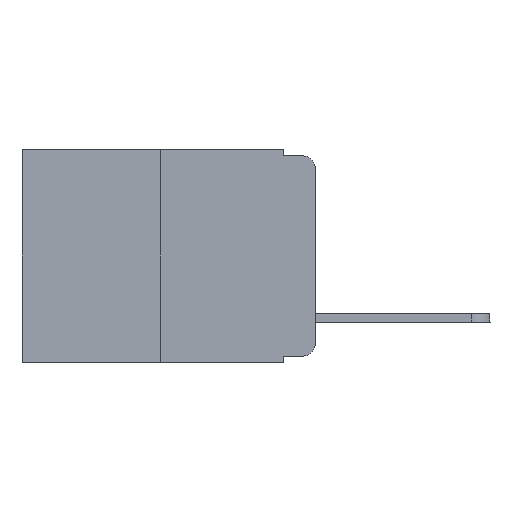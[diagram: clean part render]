
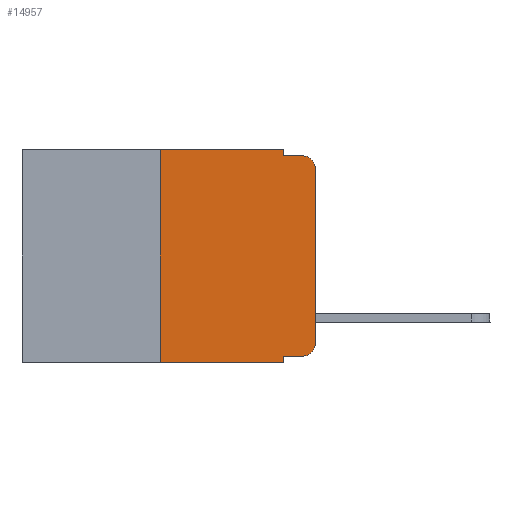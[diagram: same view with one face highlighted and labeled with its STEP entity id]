
A CAD part, left-side view. The second image highlights one B-rep face of the part: STEP entity #14957.
In plain terms, the highlighted planar face has unit normal (-1, 0, 0).
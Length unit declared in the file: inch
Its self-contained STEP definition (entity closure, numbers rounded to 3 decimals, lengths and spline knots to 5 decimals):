
#62 = DIRECTION ( 'NONE',  ( -1., 0., 0. ) ) ;
#193 = VECTOR ( 'NONE', #1713, 39.37008 ) ;
#206 = CIRCLE ( 'NONE', #14292, 0.02 ) ;
#328 = CARTESIAN_POINT ( 'NONE',  ( 0., 0.051, 0. ) ) ;
#386 = ORIENTED_EDGE ( 'NONE', *, *, #7554, .T. ) ;
#528 = VERTEX_POINT ( 'NONE', #17079 ) ;
#623 = VERTEX_POINT ( 'NONE', #13996 ) ;
#655 = VERTEX_POINT ( 'NONE', #3853 ) ;
#1291 = CARTESIAN_POINT ( 'NONE',  ( 0., 0.051, -0.01 ) ) ;
#1430 = DIRECTION ( 'NONE',  ( 0., 0., -1. ) ) ;
#1540 = VERTEX_POINT ( 'NONE', #9030 ) ;
#1619 = EDGE_CURVE ( 'NONE', #16990, #623, #7674, .T. ) ;
#1698 = VERTEX_POINT ( 'NONE', #9258 ) ;
#1713 = DIRECTION ( 'NONE',  ( 0., -1., 0. ) ) ;
#1987 = LINE ( 'NONE', #1291, #3658 ) ;
#2120 = ORIENTED_EDGE ( 'NONE', *, *, #9047, .T. ) ;
#2159 = DIRECTION ( 'NONE',  ( 0., -1., 0. ) ) ;
#2180 = ORIENTED_EDGE ( 'NONE', *, *, #7322, .T. ) ;
#2608 = CARTESIAN_POINT ( 'NONE',  ( 0., 0.051, -0.343 ) ) ;
#2778 = AXIS2_PLACEMENT_3D ( 'NONE', #9251, #13222, #5307 ) ;
#3658 = VECTOR ( 'NONE', #7928, 39.37008 ) ;
#3849 = DIRECTION ( 'NONE',  ( 0., 0., 1. ) ) ;
#3853 = CARTESIAN_POINT ( 'NONE',  ( 0., 0.02, -0.01 ) ) ;
#4006 = EDGE_CURVE ( 'NONE', #15009, #11115, #6729, .T. ) ;
#4108 = CARTESIAN_POINT ( 'NONE',  ( 0., 0.051, -0.333 ) ) ;
#4257 = EDGE_CURVE ( 'NONE', #15009, #1698, #11342, .T. ) ;
#4391 = EDGE_CURVE ( 'NONE', #1698, #16990, #13694, .T. ) ;
#4654 = FACE_OUTER_BOUND ( 'NONE', #6799, .T. ) ;
#4686 = CARTESIAN_POINT ( 'NONE',  ( 0., 0.473, -0.343 ) ) ;
#5002 = DIRECTION ( 'NONE',  ( -1., 0., 0. ) ) ;
#5216 = ORIENTED_EDGE ( 'NONE', *, *, #4257, .F. ) ;
#5307 = DIRECTION ( 'NONE',  ( 0., 0., -1. ) ) ;
#5318 = EDGE_CURVE ( 'NONE', #623, #655, #1987, .T. ) ;
#5366 = EDGE_CURVE ( 'NONE', #11737, #11115, #6347, .T. ) ;
#5807 = VECTOR ( 'NONE', #3849, 39.37008 ) ;
#6042 = CARTESIAN_POINT ( 'NONE',  ( 0., 0.473, 0. ) ) ;
#6225 = DIRECTION ( 'NONE',  ( 0., 0., -1. ) ) ;
#6347 = LINE ( 'NONE', #14552, #16394 ) ;
#6536 = CARTESIAN_POINT ( 'NONE',  ( 0., 0.25, -0.343 ) ) ;
#6538 = DIRECTION ( 'NONE',  ( 0., 0., -1. ) ) ;
#6553 = ORIENTED_EDGE ( 'NONE', *, *, #1619, .F. ) ;
#6729 = LINE ( 'NONE', #4686, #7151 ) ;
#6799 = EDGE_LOOP ( 'NONE', ( #2120, #11774, #15405, #6553, #13322, #5216, #14382, #9558, #386, #2180 ) ) ;
#7151 = VECTOR ( 'NONE', #2159, 39.37008 ) ;
#7322 = EDGE_CURVE ( 'NONE', #528, #14368, #206, .T. ) ;
#7364 = VECTOR ( 'NONE', #13797, 39.37008 ) ;
#7495 = CARTESIAN_POINT ( 'NONE',  ( 0., 0.02, -0.03 ) ) ;
#7554 = EDGE_CURVE ( 'NONE', #11737, #528, #7711, .T. ) ;
#7674 = LINE ( 'NONE', #8975, #11228 ) ;
#7711 = LINE ( 'NONE', #14980, #193 ) ;
#7834 = DIRECTION ( 'NONE',  ( 0., -1., 0. ) ) ;
#7928 = DIRECTION ( 'NONE',  ( 0., -1., 0. ) ) ;
#8975 = CARTESIAN_POINT ( 'NONE',  ( 0., 0.051, 0. ) ) ;
#9030 = CARTESIAN_POINT ( 'NONE',  ( 0., 0., -0.03 ) ) ;
#9047 = EDGE_CURVE ( 'NONE', #14368, #1540, #13302, .T. ) ;
#9251 = CARTESIAN_POINT ( 'NONE',  ( 0., 0.473, 0. ) ) ;
#9258 = CARTESIAN_POINT ( 'NONE',  ( 0., 0.25, 0. ) ) ;
#9558 = ORIENTED_EDGE ( 'NONE', *, *, #5366, .F. ) ;
#10570 = VECTOR ( 'NONE', #7834, 39.37008 ) ;
#10583 = CARTESIAN_POINT ( 'NONE',  ( 0., 0.02, -0.313 ) ) ;
#11115 = VERTEX_POINT ( 'NONE', #2608 ) ;
#11228 = VECTOR ( 'NONE', #13114, 39.37008 ) ;
#11342 = LINE ( 'NONE', #16275, #7364 ) ;
#11682 = CIRCLE ( 'NONE', #14581, 0.02 ) ;
#11737 = VERTEX_POINT ( 'NONE', #4108 ) ;
#11774 = ORIENTED_EDGE ( 'NONE', *, *, #17228, .T. ) ;
#13114 = DIRECTION ( 'NONE',  ( 0., 0., -1. ) ) ;
#13222 = DIRECTION ( 'NONE',  ( 1., 0., 0. ) ) ;
#13302 = LINE ( 'NONE', #16104, #5807 ) ;
#13322 = ORIENTED_EDGE ( 'NONE', *, *, #4391, .F. ) ;
#13694 = LINE ( 'NONE', #6042, #10570 ) ;
#13797 = DIRECTION ( 'NONE',  ( 0., 0., 1. ) ) ;
#13996 = CARTESIAN_POINT ( 'NONE',  ( 0., 0.051, -0.01 ) ) ;
#14292 = AXIS2_PLACEMENT_3D ( 'NONE', #10583, #62, #1430 ) ;
#14368 = VERTEX_POINT ( 'NONE', #15568 ) ;
#14382 = ORIENTED_EDGE ( 'NONE', *, *, #4006, .T. ) ;
#14552 = CARTESIAN_POINT ( 'NONE',  ( 0., 0.051, 0. ) ) ;
#14581 = AXIS2_PLACEMENT_3D ( 'NONE', #7495, #5002, #6225 ) ;
#14957 = ADVANCED_FACE ( 'NONE', ( #4654 ), #16906, .F. ) ;
#14980 = CARTESIAN_POINT ( 'NONE',  ( 0., 0.051, -0.333 ) ) ;
#15009 = VERTEX_POINT ( 'NONE', #6536 ) ;
#15405 = ORIENTED_EDGE ( 'NONE', *, *, #5318, .F. ) ;
#15568 = CARTESIAN_POINT ( 'NONE',  ( 0., 0., -0.313 ) ) ;
#16104 = CARTESIAN_POINT ( 'NONE',  ( 0., 0., 0. ) ) ;
#16275 = CARTESIAN_POINT ( 'NONE',  ( 0., 0.25, 0. ) ) ;
#16394 = VECTOR ( 'NONE', #6538, 39.37008 ) ;
#16906 = PLANE ( 'NONE',  #2778 ) ;
#16990 = VERTEX_POINT ( 'NONE', #328 ) ;
#17079 = CARTESIAN_POINT ( 'NONE',  ( 0., 0.02, -0.333 ) ) ;
#17228 = EDGE_CURVE ( 'NONE', #1540, #655, #11682, .T. ) ;
